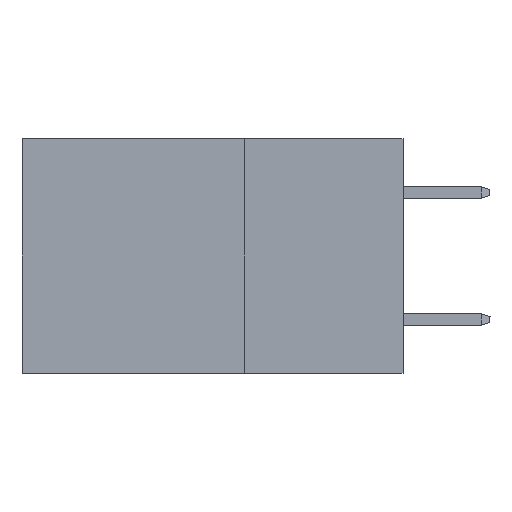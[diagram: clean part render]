
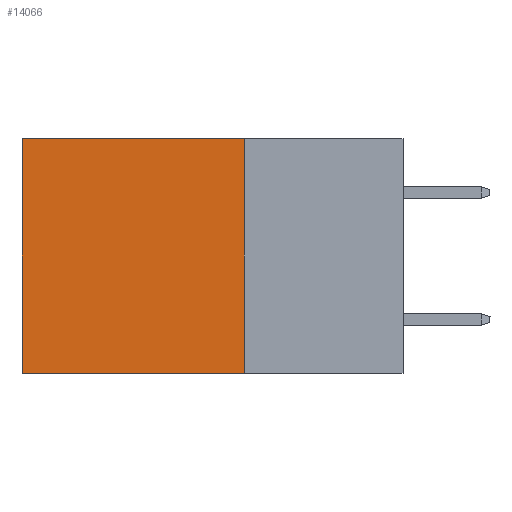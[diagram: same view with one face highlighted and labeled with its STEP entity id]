
A CAD part, left-side view. The second image highlights one B-rep face of the part: STEP entity #14066.
In plain terms, the highlighted planar face has unit normal (-1, 0, 0).
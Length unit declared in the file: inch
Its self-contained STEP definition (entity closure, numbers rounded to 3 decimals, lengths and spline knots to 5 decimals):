
#1419 = CARTESIAN_POINT ( 'NONE',  ( 0.2875, 0.6, 0. ) ) ;
#2122 = CARTESIAN_POINT ( 'NONE',  ( 0.2875, 0.6, 0. ) ) ;
#2963 = ORIENTED_EDGE ( 'NONE', *, *, #14174, .F. ) ;
#3005 = ORIENTED_EDGE ( 'NONE', *, *, #10396, .T. ) ;
#3289 = VERTEX_POINT ( 'NONE', #9641 ) ;
#3896 = CARTESIAN_POINT ( 'NONE',  ( 0.2875, 0.25, -0.37 ) ) ;
#3922 = CARTESIAN_POINT ( 'NONE',  ( 0.2875, 0.25, 0. ) ) ;
#4781 = VECTOR ( 'NONE', #17990, 39.37008 ) ;
#6087 = DIRECTION ( 'NONE',  ( 0., 0., -1. ) ) ;
#6980 = VECTOR ( 'NONE', #10384, 39.37008 ) ;
#7415 = CARTESIAN_POINT ( 'NONE',  ( 0.2875, 0.25, 0. ) ) ;
#7580 = ORIENTED_EDGE ( 'NONE', *, *, #14284, .T. ) ;
#8640 = LINE ( 'NONE', #3896, #4781 ) ;
#9641 = CARTESIAN_POINT ( 'NONE',  ( 0.2875, 0.25, 0. ) ) ;
#9750 = FACE_OUTER_BOUND ( 'NONE', #18121, .T. ) ;
#10384 = DIRECTION ( 'NONE',  ( 0., 0., -1. ) ) ;
#10396 = EDGE_CURVE ( 'NONE', #19855, #12173, #18557, .T. ) ;
#11070 = CARTESIAN_POINT ( 'NONE',  ( 0.2875, 0.25, 0. ) ) ;
#11176 = EDGE_CURVE ( 'NONE', #3289, #13327, #11591, .T. ) ;
#11591 = LINE ( 'NONE', #3922, #6980 ) ;
#12169 = AXIS2_PLACEMENT_3D ( 'NONE', #11070, #18713, #15823 ) ;
#12173 = VERTEX_POINT ( 'NONE', #16625 ) ;
#13327 = VERTEX_POINT ( 'NONE', #14684 ) ;
#13742 = VECTOR ( 'NONE', #6087, 39.37008 ) ;
#13881 = DIRECTION ( 'NONE',  ( 0., 1., 0. ) ) ;
#14066 = ADVANCED_FACE ( 'NONE', ( #9750 ), #17264, .F. ) ;
#14114 = VECTOR ( 'NONE', #13881, 39.37008 ) ;
#14174 = EDGE_CURVE ( 'NONE', #13327, #12173, #8640, .T. ) ;
#14284 = EDGE_CURVE ( 'NONE', #3289, #19855, #18393, .T. ) ;
#14684 = CARTESIAN_POINT ( 'NONE',  ( 0.2875, 0.25, -0.37 ) ) ;
#15823 = DIRECTION ( 'NONE',  ( 0., 0., -1. ) ) ;
#16625 = CARTESIAN_POINT ( 'NONE',  ( 0.2875, 0.6, -0.37 ) ) ;
#17264 = PLANE ( 'NONE',  #12169 ) ;
#17990 = DIRECTION ( 'NONE',  ( 0., 1., 0. ) ) ;
#18121 = EDGE_LOOP ( 'NONE', ( #3005, #2963, #18452, #7580 ) ) ;
#18393 = LINE ( 'NONE', #7415, #14114 ) ;
#18452 = ORIENTED_EDGE ( 'NONE', *, *, #11176, .F. ) ;
#18557 = LINE ( 'NONE', #1419, #13742 ) ;
#18713 = DIRECTION ( 'NONE',  ( 1., 0., 0. ) ) ;
#19855 = VERTEX_POINT ( 'NONE', #2122 ) ;
